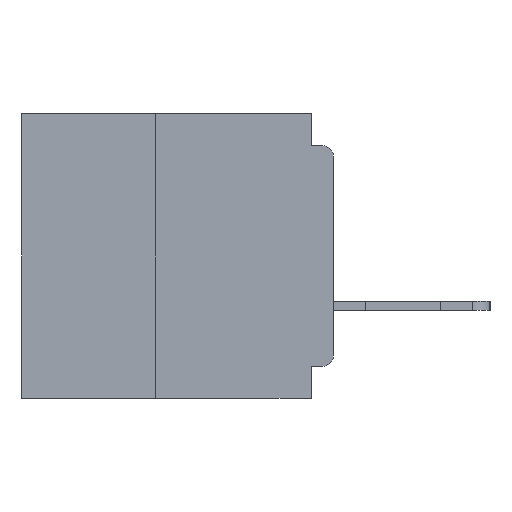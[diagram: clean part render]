
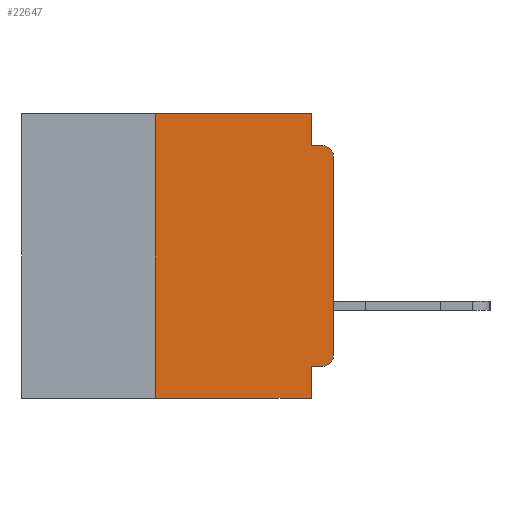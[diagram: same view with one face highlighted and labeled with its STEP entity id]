
A CAD part, left-side view. The second image highlights one B-rep face of the part: STEP entity #22647.
In plain terms, the highlighted planar face has unit normal (-1, 0, 0).
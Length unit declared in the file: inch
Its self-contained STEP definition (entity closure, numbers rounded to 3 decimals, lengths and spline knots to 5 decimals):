
#245 = AXIS2_PLACEMENT_3D ( 'NONE', #26441, #26428, #26396 ) ;
#1690 = CARTESIAN_POINT ( 'NONE',  ( 0., 0.031, 0. ) ) ;
#2167 = CARTESIAN_POINT ( 'NONE',  ( 0., 0., -0.045 ) ) ;
#3009 = VERTEX_POINT ( 'NONE', #31897 ) ;
#3085 = VECTOR ( 'NONE', #32479, 39.37008 ) ;
#3576 = CARTESIAN_POINT ( 'NONE',  ( 0., 0.437, 0. ) ) ;
#3683 = CARTESIAN_POINT ( 'NONE',  ( 0., 0., -0.34 ) ) ;
#3789 = VERTEX_POINT ( 'NONE', #33926 ) ;
#3812 = ORIENTED_EDGE ( 'NONE', *, *, #17201, .F. ) ;
#4105 = VECTOR ( 'NONE', #18303, 39.37008 ) ;
#4777 = VECTOR ( 'NONE', #5117, 39.37008 ) ;
#4962 = ORIENTED_EDGE ( 'NONE', *, *, #19698, .F. ) ;
#5114 = AXIS2_PLACEMENT_3D ( 'NONE', #3576, #28493, #11944 ) ;
#5117 = DIRECTION ( 'NONE',  ( 0., -1., 0. ) ) ;
#5344 = EDGE_CURVE ( 'NONE', #9953, #25254, #25266, .T. ) ;
#5789 = VERTEX_POINT ( 'NONE', #8873 ) ;
#5919 = CIRCLE ( 'NONE', #14539, 0.015 ) ;
#6088 = DIRECTION ( 'NONE',  ( -1., 0., 0. ) ) ;
#7231 = ORIENTED_EDGE ( 'NONE', *, *, #29368, .F. ) ;
#8177 = CARTESIAN_POINT ( 'NONE',  ( 0., 0.437, 0. ) ) ;
#8278 = CARTESIAN_POINT ( 'NONE',  ( 0., 0., -0.06 ) ) ;
#8325 = ORIENTED_EDGE ( 'NONE', *, *, #15021, .T. ) ;
#8873 = CARTESIAN_POINT ( 'NONE',  ( 0., 0.031, -0.045 ) ) ;
#8879 = VECTOR ( 'NONE', #13066, 39.37008 ) ;
#9953 = VERTEX_POINT ( 'NONE', #8278 ) ;
#10279 = CARTESIAN_POINT ( 'NONE',  ( 0., 0., -0.355 ) ) ;
#10489 = LINE ( 'NONE', #15990, #3085 ) ;
#10875 = EDGE_LOOP ( 'NONE', ( #8325, #28816, #25836, #30525, #7231, #32910, #34147, #4962, #3812, #29220 ) ) ;
#11445 = VERTEX_POINT ( 'NONE', #23779 ) ;
#11644 = LINE ( 'NONE', #25069, #32789 ) ;
#11944 = DIRECTION ( 'NONE',  ( 0., 0., -1. ) ) ;
#12897 = CARTESIAN_POINT ( 'NONE',  ( 0., 0.031, -0.4 ) ) ;
#13066 = DIRECTION ( 'NONE',  ( 0., 1., 0. ) ) ;
#13141 = DIRECTION ( 'NONE',  ( 0., 0., 1. ) ) ;
#13223 = LINE ( 'NONE', #31982, #4105 ) ;
#14539 = AXIS2_PLACEMENT_3D ( 'NONE', #22679, #6088, #25444 ) ;
#15021 = EDGE_CURVE ( 'NONE', #29028, #9953, #11644, .T. ) ;
#15990 = CARTESIAN_POINT ( 'NONE',  ( 0., 0.031, 0. ) ) ;
#16267 = LINE ( 'NONE', #10279, #8879 ) ;
#16795 = VECTOR ( 'NONE', #24762, 39.37008 ) ;
#16917 = CARTESIAN_POINT ( 'NONE',  ( 0., 0.031, -0.4 ) ) ;
#17139 = EDGE_CURVE ( 'NONE', #3789, #32800, #13223, .T. ) ;
#17201 = EDGE_CURVE ( 'NONE', #11445, #3009, #16267, .T. ) ;
#17668 = LINE ( 'NONE', #8177, #16795 ) ;
#18303 = DIRECTION ( 'NONE',  ( 0., -1., 0. ) ) ;
#18881 = EDGE_CURVE ( 'NONE', #24424, #5789, #10489, .T. ) ;
#19156 = VECTOR ( 'NONE', #33489, 39.37008 ) ;
#19698 = EDGE_CURVE ( 'NONE', #3009, #32800, #33764, .T. ) ;
#21422 = VERTEX_POINT ( 'NONE', #31326 ) ;
#21486 = CARTESIAN_POINT ( 'NONE',  ( 0., 0.25, -0.4 ) ) ;
#22473 = VECTOR ( 'NONE', #13141, 39.37008 ) ;
#22647 = ADVANCED_FACE ( 'NONE', ( #26077 ), #33897, .F. ) ;
#22679 = CARTESIAN_POINT ( 'NONE',  ( 0., 0.015, -0.34 ) ) ;
#23340 = LINE ( 'NONE', #21486, #22473 ) ;
#23779 = CARTESIAN_POINT ( 'NONE',  ( 0., 0.015, -0.355 ) ) ;
#24424 = VERTEX_POINT ( 'NONE', #1690 ) ;
#24490 = EDGE_CURVE ( 'NONE', #3789, #21422, #23340, .T. ) ;
#24762 = DIRECTION ( 'NONE',  ( 0., -1., 0. ) ) ;
#25069 = CARTESIAN_POINT ( 'NONE',  ( 0., 0., 0. ) ) ;
#25254 = VERTEX_POINT ( 'NONE', #27583 ) ;
#25266 = CIRCLE ( 'NONE', #245, 0.015 ) ;
#25444 = DIRECTION ( 'NONE',  ( 0., 0., -1. ) ) ;
#25836 = ORIENTED_EDGE ( 'NONE', *, *, #27597, .F. ) ;
#26077 = FACE_OUTER_BOUND ( 'NONE', #10875, .T. ) ;
#26396 = DIRECTION ( 'NONE',  ( 0., 0., -1. ) ) ;
#26428 = DIRECTION ( 'NONE',  ( -1., 0., 0. ) ) ;
#26441 = CARTESIAN_POINT ( 'NONE',  ( 0., 0.015, -0.06 ) ) ;
#27583 = CARTESIAN_POINT ( 'NONE',  ( 0., 0.015, -0.045 ) ) ;
#27597 = EDGE_CURVE ( 'NONE', #5789, #25254, #34140, .T. ) ;
#28493 = DIRECTION ( 'NONE',  ( 1., 0., 0. ) ) ;
#28816 = ORIENTED_EDGE ( 'NONE', *, *, #5344, .T. ) ;
#29028 = VERTEX_POINT ( 'NONE', #3683 ) ;
#29220 = ORIENTED_EDGE ( 'NONE', *, *, #29521, .T. ) ;
#29368 = EDGE_CURVE ( 'NONE', #21422, #24424, #17668, .T. ) ;
#29521 = EDGE_CURVE ( 'NONE', #11445, #29028, #5919, .T. ) ;
#30525 = ORIENTED_EDGE ( 'NONE', *, *, #18881, .F. ) ;
#30556 = DIRECTION ( 'NONE',  ( 0., 0., 1. ) ) ;
#31326 = CARTESIAN_POINT ( 'NONE',  ( 0., 0.25, 0. ) ) ;
#31897 = CARTESIAN_POINT ( 'NONE',  ( 0., 0.031, -0.355 ) ) ;
#31982 = CARTESIAN_POINT ( 'NONE',  ( 0., 0.437, -0.4 ) ) ;
#32479 = DIRECTION ( 'NONE',  ( 0., 0., -1. ) ) ;
#32789 = VECTOR ( 'NONE', #30556, 39.37008 ) ;
#32800 = VERTEX_POINT ( 'NONE', #12897 ) ;
#32910 = ORIENTED_EDGE ( 'NONE', *, *, #24490, .F. ) ;
#33489 = DIRECTION ( 'NONE',  ( 0., 0., -1. ) ) ;
#33764 = LINE ( 'NONE', #16917, #19156 ) ;
#33897 = PLANE ( 'NONE',  #5114 ) ;
#33926 = CARTESIAN_POINT ( 'NONE',  ( 0., 0.25, -0.4 ) ) ;
#34140 = LINE ( 'NONE', #2167, #4777 ) ;
#34147 = ORIENTED_EDGE ( 'NONE', *, *, #17139, .T. ) ;
